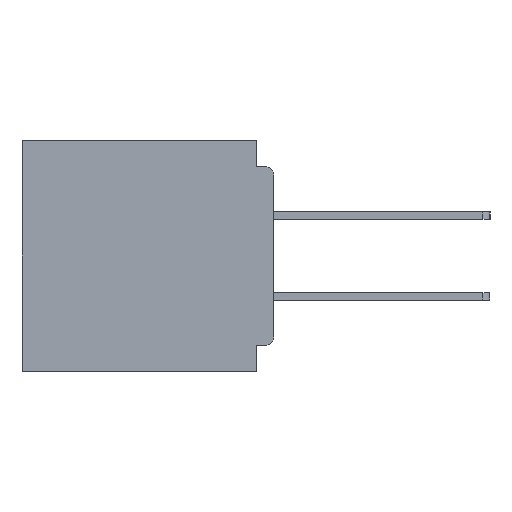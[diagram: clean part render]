
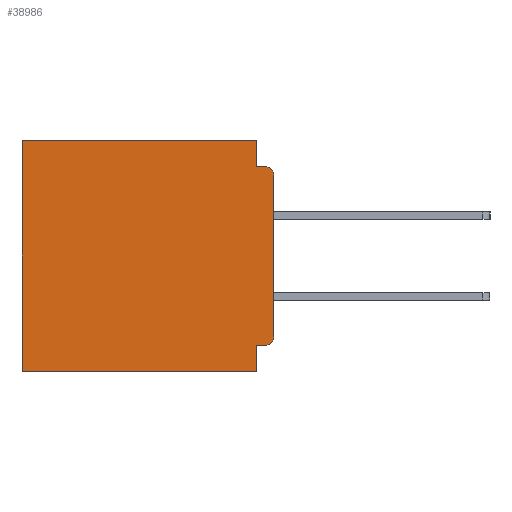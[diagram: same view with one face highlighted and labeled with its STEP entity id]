
A CAD part, left-side view. The second image highlights one B-rep face of the part: STEP entity #38986.
In plain terms, the highlighted planar face has unit normal (-1, 0, 0).
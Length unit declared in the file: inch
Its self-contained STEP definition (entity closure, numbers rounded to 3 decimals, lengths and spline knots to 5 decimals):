
#906 = CARTESIAN_POINT ( 'NONE',  ( 0.3, 0.031, -0.4 ) ) ;
#1738 = LINE ( 'NONE', #55466, #49181 ) ;
#2279 = CARTESIAN_POINT ( 'NONE',  ( 0.3, 0.437, -0.4 ) ) ;
#2433 = CARTESIAN_POINT ( 'NONE',  ( 0.3, 0., -0.34 ) ) ;
#4217 = DIRECTION ( 'NONE',  ( 0., 0., -1. ) ) ;
#5493 = VECTOR ( 'NONE', #17043, 39.37008 ) ;
#5697 = EDGE_CURVE ( 'NONE', #14871, #45395, #59710, .T. ) ;
#6529 = EDGE_CURVE ( 'NONE', #44004, #45395, #26457, .T. ) ;
#6689 = EDGE_LOOP ( 'NONE', ( #56762, #28982, #21717, #8119, #50435, #7703, #29759, #22006, #27825, #7817 ) ) ;
#6707 = AXIS2_PLACEMENT_3D ( 'NONE', #55568, #27271, #60220 ) ;
#7308 = DIRECTION ( 'NONE',  ( 0., 0., -1. ) ) ;
#7429 = VECTOR ( 'NONE', #47688, 39.37008 ) ;
#7703 = ORIENTED_EDGE ( 'NONE', *, *, #13590, .T. ) ;
#7817 = ORIENTED_EDGE ( 'NONE', *, *, #53682, .T. ) ;
#7909 = LINE ( 'NONE', #60285, #55278 ) ;
#8119 = ORIENTED_EDGE ( 'NONE', *, *, #35358, .F. ) ;
#8771 = VERTEX_POINT ( 'NONE', #906 ) ;
#10691 = VERTEX_POINT ( 'NONE', #38886 ) ;
#12056 = EDGE_CURVE ( 'NONE', #44004, #28676, #1738, .T. ) ;
#13507 = VECTOR ( 'NONE', #38144, 39.37008 ) ;
#13590 = EDGE_CURVE ( 'NONE', #32487, #42001, #40162, .T. ) ;
#13873 = FACE_OUTER_BOUND ( 'NONE', #6689, .T. ) ;
#14871 = VERTEX_POINT ( 'NONE', #53434 ) ;
#14873 = CARTESIAN_POINT ( 'NONE',  ( 0.3, 0.015, -0.355 ) ) ;
#16649 = DIRECTION ( 'NONE',  ( 0., 1., 0. ) ) ;
#17043 = DIRECTION ( 'NONE',  ( 0., 1., 0. ) ) ;
#17657 = VECTOR ( 'NONE', #16649, 39.37008 ) ;
#17708 = DIRECTION ( 'NONE',  ( 0., 0., -1. ) ) ;
#18457 = CARTESIAN_POINT ( 'NONE',  ( 0.3, 0., -0.4 ) ) ;
#20162 = LINE ( 'NONE', #24245, #7429 ) ;
#21717 = ORIENTED_EDGE ( 'NONE', *, *, #5697, .F. ) ;
#22006 = ORIENTED_EDGE ( 'NONE', *, *, #50234, .F. ) ;
#22602 = AXIS2_PLACEMENT_3D ( 'NONE', #22913, #55911, #27634 ) ;
#22913 = CARTESIAN_POINT ( 'NONE',  ( 0.3, 0.015, -0.34 ) ) ;
#24245 = CARTESIAN_POINT ( 'NONE',  ( 0.3, 0.031, 0. ) ) ;
#25992 = VECTOR ( 'NONE', #7308, 39.37008 ) ;
#26457 = CIRCLE ( 'NONE', #6707, 0.015 ) ;
#27271 = DIRECTION ( 'NONE',  ( -1., 0., 0. ) ) ;
#27634 = DIRECTION ( 'NONE',  ( 0., 0., -1. ) ) ;
#27825 = ORIENTED_EDGE ( 'NONE', *, *, #32722, .F. ) ;
#28676 = VERTEX_POINT ( 'NONE', #2433 ) ;
#28982 = ORIENTED_EDGE ( 'NONE', *, *, #6529, .T. ) ;
#29759 = ORIENTED_EDGE ( 'NONE', *, *, #54119, .F. ) ;
#31053 = CARTESIAN_POINT ( 'NONE',  ( 0.3, 0., 0. ) ) ;
#32487 = VERTEX_POINT ( 'NONE', #49243 ) ;
#32664 = DIRECTION ( 'NONE',  ( 1., 0., 0. ) ) ;
#32722 = EDGE_CURVE ( 'NONE', #53243, #10691, #7909, .T. ) ;
#33673 = LINE ( 'NONE', #31053, #5493 ) ;
#35358 = EDGE_CURVE ( 'NONE', #51693, #14871, #20162, .T. ) ;
#38144 = DIRECTION ( 'NONE',  ( 0., 0., -1. ) ) ;
#38886 = CARTESIAN_POINT ( 'NONE',  ( 0.3, 0.031, -0.355 ) ) ;
#38986 = ADVANCED_FACE ( 'NONE', ( #13873 ), #60872, .F. ) ;
#39872 = CIRCLE ( 'NONE', #22602, 0.015 ) ;
#40002 = LINE ( 'NONE', #40477, #25992 ) ;
#40162 = LINE ( 'NONE', #42916, #13507 ) ;
#40187 = CARTESIAN_POINT ( 'NONE',  ( 0.3, 0., -0.4 ) ) ;
#40477 = CARTESIAN_POINT ( 'NONE',  ( 0.3, 0.031, -0.4 ) ) ;
#40904 = EDGE_CURVE ( 'NONE', #51693, #32487, #33673, .T. ) ;
#42001 = VERTEX_POINT ( 'NONE', #2279 ) ;
#42916 = CARTESIAN_POINT ( 'NONE',  ( 0.3, 0.437, -0.4 ) ) ;
#44004 = VERTEX_POINT ( 'NONE', #56030 ) ;
#45395 = VERTEX_POINT ( 'NONE', #52398 ) ;
#45697 = LINE ( 'NONE', #40187, #17657 ) ;
#46300 = DIRECTION ( 'NONE',  ( 0., 1., 0. ) ) ;
#46626 = AXIS2_PLACEMENT_3D ( 'NONE', #18457, #32664, #4217 ) ;
#47173 = VECTOR ( 'NONE', #58935, 39.37008 ) ;
#47688 = DIRECTION ( 'NONE',  ( 0., 0., -1. ) ) ;
#49181 = VECTOR ( 'NONE', #17708, 39.37008 ) ;
#49239 = CARTESIAN_POINT ( 'NONE',  ( 0.3, 0., -0.045 ) ) ;
#49243 = CARTESIAN_POINT ( 'NONE',  ( 0.3, 0.437, 0. ) ) ;
#50234 = EDGE_CURVE ( 'NONE', #10691, #8771, #40002, .T. ) ;
#50435 = ORIENTED_EDGE ( 'NONE', *, *, #40904, .T. ) ;
#51693 = VERTEX_POINT ( 'NONE', #59986 ) ;
#52398 = CARTESIAN_POINT ( 'NONE',  ( 0.3, 0.015, -0.045 ) ) ;
#53243 = VERTEX_POINT ( 'NONE', #14873 ) ;
#53434 = CARTESIAN_POINT ( 'NONE',  ( 0.3, 0.031, -0.045 ) ) ;
#53682 = EDGE_CURVE ( 'NONE', #53243, #28676, #39872, .T. ) ;
#54119 = EDGE_CURVE ( 'NONE', #8771, #42001, #45697, .T. ) ;
#55278 = VECTOR ( 'NONE', #46300, 39.37008 ) ;
#55466 = CARTESIAN_POINT ( 'NONE',  ( 0.3, 0., -0.4 ) ) ;
#55568 = CARTESIAN_POINT ( 'NONE',  ( 0.3, 0.015, -0.06 ) ) ;
#55911 = DIRECTION ( 'NONE',  ( -1., 0., 0. ) ) ;
#56030 = CARTESIAN_POINT ( 'NONE',  ( 0.3, 0., -0.06 ) ) ;
#56762 = ORIENTED_EDGE ( 'NONE', *, *, #12056, .F. ) ;
#58935 = DIRECTION ( 'NONE',  ( 0., -1., 0. ) ) ;
#59710 = LINE ( 'NONE', #49239, #47173 ) ;
#59986 = CARTESIAN_POINT ( 'NONE',  ( 0.3, 0.031, 0. ) ) ;
#60220 = DIRECTION ( 'NONE',  ( 0., 0., -1. ) ) ;
#60285 = CARTESIAN_POINT ( 'NONE',  ( 0.3, 0., -0.355 ) ) ;
#60872 = PLANE ( 'NONE',  #46626 ) ;
